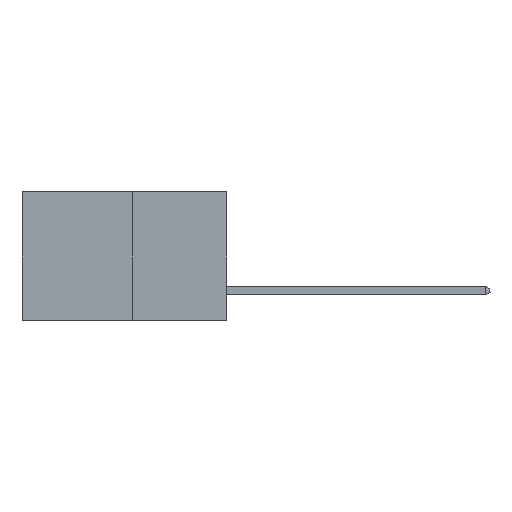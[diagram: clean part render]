
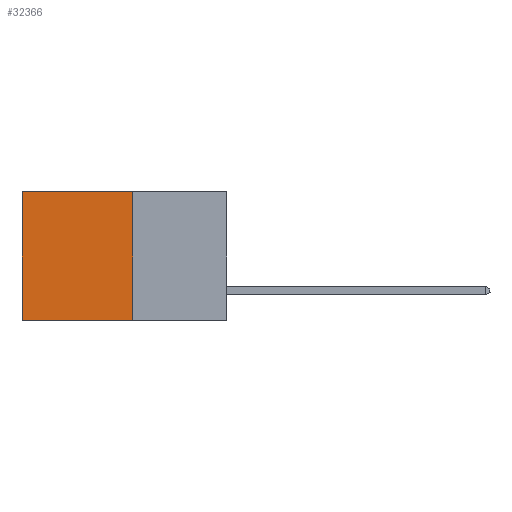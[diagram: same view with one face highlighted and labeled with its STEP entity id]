
A CAD part, left-side view. The second image highlights one B-rep face of the part: STEP entity #32366.
In plain terms, the highlighted planar face has unit normal (-1, 0, 0).
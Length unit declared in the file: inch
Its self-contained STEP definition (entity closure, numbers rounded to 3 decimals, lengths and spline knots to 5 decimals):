
#1167 = CARTESIAN_POINT ( 'NONE',  ( 0.277, 0.27, 0. ) ) ;
#1429 = CARTESIAN_POINT ( 'NONE',  ( 0.277, 0.59, 0. ) ) ;
#1716 = VERTEX_POINT ( 'NONE', #16077 ) ;
#2607 = CARTESIAN_POINT ( 'NONE',  ( 0.277, 0.27, -0.37 ) ) ;
#3459 = CARTESIAN_POINT ( 'NONE',  ( 0.277, 0.27, 0. ) ) ;
#3880 = DIRECTION ( 'NONE',  ( 0., 1., 0. ) ) ;
#4661 = LINE ( 'NONE', #26703, #17827 ) ;
#5095 = DIRECTION ( 'NONE',  ( 1., 0., 0. ) ) ;
#5447 = DIRECTION ( 'NONE',  ( 0., 0., -1. ) ) ;
#5884 = VERTEX_POINT ( 'NONE', #30339 ) ;
#6948 = AXIS2_PLACEMENT_3D ( 'NONE', #20868, #5095, #23644 ) ;
#6975 = VECTOR ( 'NONE', #3880, 39.37008 ) ;
#7567 = EDGE_LOOP ( 'NONE', ( #13834, #28288, #15142, #30363 ) ) ;
#9713 = LINE ( 'NONE', #2607, #30926 ) ;
#13007 = DIRECTION ( 'NONE',  ( 0., 0., -1. ) ) ;
#13834 = ORIENTED_EDGE ( 'NONE', *, *, #15827, .T. ) ;
#14838 = VERTEX_POINT ( 'NONE', #3459 ) ;
#15142 = ORIENTED_EDGE ( 'NONE', *, *, #17048, .F. ) ;
#15544 = PLANE ( 'NONE',  #6948 ) ;
#15827 = EDGE_CURVE ( 'NONE', #21923, #1716, #4661, .T. ) ;
#16077 = CARTESIAN_POINT ( 'NONE',  ( 0.277, 0.59, -0.37 ) ) ;
#17048 = EDGE_CURVE ( 'NONE', #14838, #5884, #33684, .T. ) ;
#17827 = VECTOR ( 'NONE', #5447, 39.37008 ) ;
#18403 = DIRECTION ( 'NONE',  ( 0., 1., 0. ) ) ;
#19343 = VECTOR ( 'NONE', #13007, 39.37008 ) ;
#20868 = CARTESIAN_POINT ( 'NONE',  ( 0.277, 0.27, -0.37 ) ) ;
#21923 = VERTEX_POINT ( 'NONE', #1429 ) ;
#23644 = DIRECTION ( 'NONE',  ( 0., 0., -1. ) ) ;
#24635 = EDGE_CURVE ( 'NONE', #14838, #21923, #27311, .T. ) ;
#26703 = CARTESIAN_POINT ( 'NONE',  ( 0.277, 0.59, -0.37 ) ) ;
#27311 = LINE ( 'NONE', #1167, #6975 ) ;
#27855 = FACE_OUTER_BOUND ( 'NONE', #7567, .T. ) ;
#28288 = ORIENTED_EDGE ( 'NONE', *, *, #28798, .F. ) ;
#28798 = EDGE_CURVE ( 'NONE', #5884, #1716, #9713, .T. ) ;
#30339 = CARTESIAN_POINT ( 'NONE',  ( 0.277, 0.27, -0.37 ) ) ;
#30363 = ORIENTED_EDGE ( 'NONE', *, *, #24635, .T. ) ;
#30926 = VECTOR ( 'NONE', #18403, 39.37008 ) ;
#31651 = CARTESIAN_POINT ( 'NONE',  ( 0.277, 0.27, -0.37 ) ) ;
#32366 = ADVANCED_FACE ( 'NONE', ( #27855 ), #15544, .F. ) ;
#33684 = LINE ( 'NONE', #31651, #19343 ) ;
